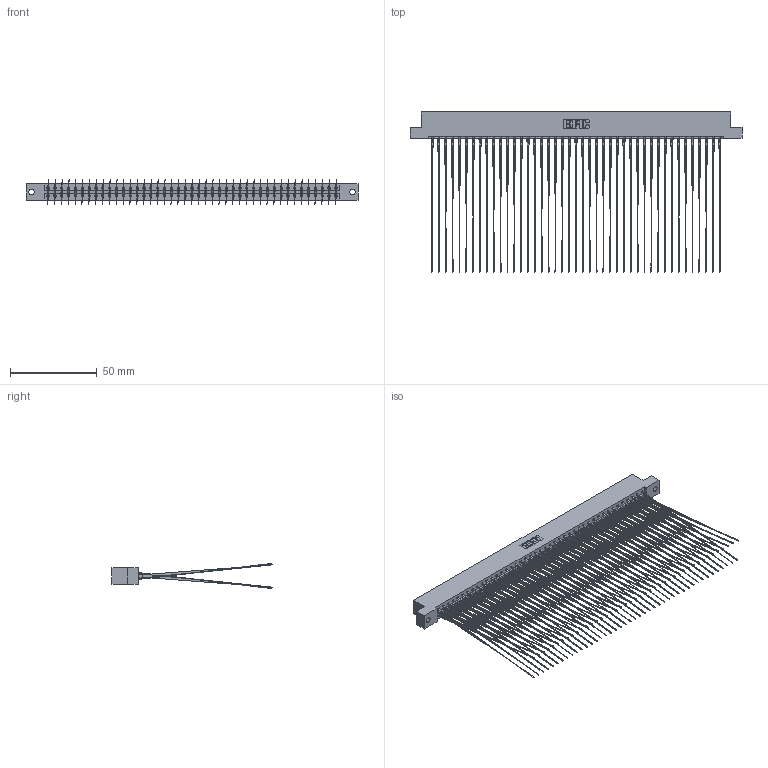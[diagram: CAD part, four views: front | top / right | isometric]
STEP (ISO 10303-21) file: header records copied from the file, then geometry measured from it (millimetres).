
FILE_DESCRIPTION (( 'STEP AP203' ), '1' );
FILE_NAME ('833-086-556-202.STEP', '2020-06-06T03:58:42', ( '' ), ( '' ), 'SwSTEP 2.0', 'SolidWorks 2020', '' );
FILE_SCHEMA (( 'CONFIG_CONTROL_DESIGN' ));
Length unit declared in the file: inch
Products named in the file (3): 833 Part_Flush - .128 Dia; 833-086-556-202; 345-292-001_556 Tail
Assembly tree (87 placements, depth 2):
  833-086-556-202
    833 Part_Flush - .128 Dia
    345-292-001_556 Tail  x86
Bounding box: 191.92 x 92.51 x 14.41 mm (x, y, z)
Volume: 20266.6 mm3; surface area: 18615.8 mm2
Topology: 87 solids, 87 shells, 5102 faces, 15189 edges, 10096 vertices
Faces by surface type: plane 3510, cylinder 1592
Entity records: 27757 total; most frequent: CARTESIAN_POINT 4614, ORIENTED_EDGE 4538, DIRECTION 3929, EDGE_CURVE 2269, VECTOR 2133, LINE 2133, VERTEX_POINT 1510, AXIS2_PLACEMENT_3D 898
